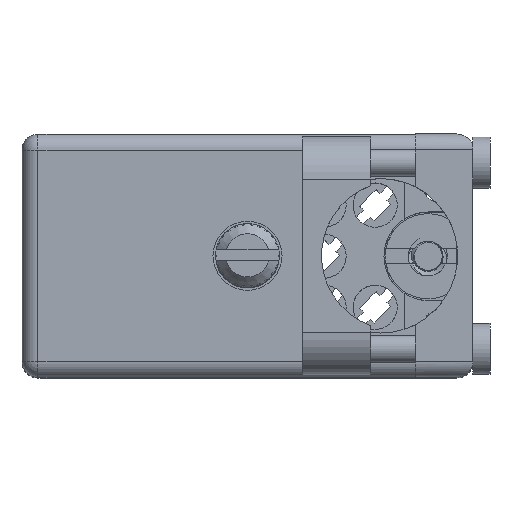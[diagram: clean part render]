
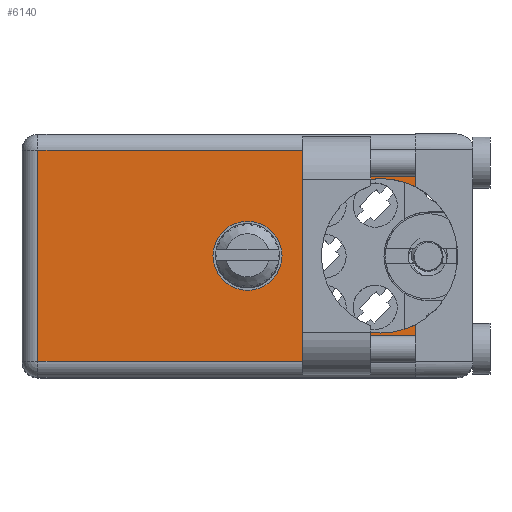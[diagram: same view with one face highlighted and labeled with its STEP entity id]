
A CAD part, top view. The second image highlights one B-rep face of the part: STEP entity #6140.
In plain terms, the highlighted face is planar.
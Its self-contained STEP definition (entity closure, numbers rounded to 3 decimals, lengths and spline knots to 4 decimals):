
#1136 = CARTESIAN_POINT ( 'NONE',  ( 1.053, 0.906, -0.3575 ) ) ;
#6140 = ADVANCED_FACE ( 'NONE', ( #109028, #7195 ), #143802, .T. ) ;
#7195 = FACE_BOUND ( 'NONE', #37577, .T. ) ;
#7939 = EDGE_CURVE ( 'NONE', #183258, #33568, #13675, .T. ) ;
#9528 = VERTEX_POINT ( 'NONE', #151142 ) ;
#9770 = DIRECTION ( 'NONE',  ( 0., 0., 1. ) ) ;
#9917 = DIRECTION ( 'NONE',  ( 0., 0., 1. ) ) ;
#13675 = CIRCLE ( 'NONE', #28924, 0.227 ) ;
#15216 = LINE ( 'NONE', #37053, #128751 ) ;
#16511 = CARTESIAN_POINT ( 'NONE',  ( 1.155, 0.906, -0.047 ) ) ;
#20116 = CIRCLE ( 'NONE', #103181, 0.1015 ) ;
#27319 = CARTESIAN_POINT ( 'NONE',  ( 1.053, 0.906, -0.3575 ) ) ;
#27502 = VERTEX_POINT ( 'NONE', #127699 ) ;
#28924 = AXIS2_PLACEMENT_3D ( 'NONE', #80984, #184537, #99670 ) ;
#32503 = VECTOR ( 'NONE', #9917, 39.3701 ) ;
#33568 = VERTEX_POINT ( 'NONE', #42407 ) ;
#33758 = VERTEX_POINT ( 'NONE', #16511 ) ;
#36084 = CARTESIAN_POINT ( 'NONE',  ( 1.155, 0.906, 0. ) ) ;
#37053 = CARTESIAN_POINT ( 'NONE',  ( 1.155, 0.906, -0.047 ) ) ;
#37577 = EDGE_LOOP ( 'NONE', ( #189435, #42426 ) ) ;
#41265 = VERTEX_POINT ( 'NONE', #84874 ) ;
#41663 = CIRCLE ( 'NONE', #69312, 0.1015 ) ;
#42241 = DIRECTION ( 'NONE',  ( 0., 0., 1. ) ) ;
#42407 = CARTESIAN_POINT ( 'NONE',  ( 1.053, 0.906, -0.1305 ) ) ;
#42426 = ORIENTED_EDGE ( 'NONE', *, *, #114683, .F. ) ;
#43009 = ORIENTED_EDGE ( 'NONE', *, *, #78092, .F. ) ;
#52280 = CARTESIAN_POINT ( 'NONE',  ( 0.6625, 0.906, -0.3575 ) ) ;
#53597 = AXIS2_PLACEMENT_3D ( 'NONE', #1136, #150107, #147504 ) ;
#53755 = VECTOR ( 'NONE', #184150, 39.3701 ) ;
#53814 = ORIENTED_EDGE ( 'NONE', *, *, #183265, .F. ) ;
#54839 = DIRECTION ( 'NONE',  ( 0., 1., 0. ) ) ;
#57196 = DIRECTION ( 'NONE',  ( 0., 1., 0. ) ) ;
#58716 = ORIENTED_EDGE ( 'NONE', *, *, #7939, .F. ) ;
#62073 = CARTESIAN_POINT ( 'NONE',  ( 1.053, 0.906, -0.5845 ) ) ;
#63415 = VERTEX_POINT ( 'NONE', #100840 ) ;
#65922 = AXIS2_PLACEMENT_3D ( 'NONE', #158731, #141915, #9770 ) ;
#69312 = AXIS2_PLACEMENT_3D ( 'NONE', #100606, #57196, #98710 ) ;
#78092 = EDGE_CURVE ( 'NONE', #116391, #183258, #175600, .T. ) ;
#80984 = CARTESIAN_POINT ( 'NONE',  ( 1.053, 0.906, -0.3575 ) ) ;
#81599 = EDGE_CURVE ( 'NONE', #63415, #41265, #140386, .T. ) ;
#84874 = CARTESIAN_POINT ( 'NONE',  ( 0.047, 0.906, -0.047 ) ) ;
#90795 = ORIENTED_EDGE ( 'NONE', *, *, #81599, .T. ) ;
#94209 = CARTESIAN_POINT ( 'NONE',  ( 0., 0.906, -0.668 ) ) ;
#98710 = DIRECTION ( 'NONE',  ( 0., 0., 1. ) ) ;
#99670 = DIRECTION ( 'NONE',  ( 0., 0., 1. ) ) ;
#100606 = CARTESIAN_POINT ( 'NONE',  ( 0.6625, 0.906, -0.3575 ) ) ;
#100840 = CARTESIAN_POINT ( 'NONE',  ( 0.047, 0.906, -0.668 ) ) ;
#103181 = AXIS2_PLACEMENT_3D ( 'NONE', #52280, #54839, #158448 ) ;
#107796 = EDGE_CURVE ( 'NONE', #9528, #63415, #183462, .T. ) ;
#109028 = FACE_OUTER_BOUND ( 'NONE', #133324, .T. ) ;
#112223 = VERTEX_POINT ( 'NONE', #140063 ) ;
#114683 = EDGE_CURVE ( 'NONE', #27502, #186043, #20116, .T. ) ;
#116391 = VERTEX_POINT ( 'NONE', #187003 ) ;
#119215 = EDGE_CURVE ( 'NONE', #186043, #27502, #41663, .T. ) ;
#120023 = VECTOR ( 'NONE', #153345, 39.3701 ) ;
#125091 = EDGE_CURVE ( 'NONE', #41265, #33758, #15216, .T. ) ;
#126519 = AXIS2_PLACEMENT_3D ( 'NONE', #27319, #130902, #42241 ) ;
#127699 = CARTESIAN_POINT ( 'NONE',  ( 0.6625, 0.906, -0.459 ) ) ;
#128741 = CARTESIAN_POINT ( 'NONE',  ( 0.047, 0.906, -0.715 ) ) ;
#128751 = VECTOR ( 'NONE', #140657, 39.3701 ) ;
#130902 = DIRECTION ( 'NONE',  ( 0., 1., 0. ) ) ;
#133324 = EDGE_LOOP ( 'NONE', ( #53814, #171525, #90795, #149166, #173152, #147024, #58716, #43009 ) ) ;
#133467 = VECTOR ( 'NONE', #146830, 39.3701 ) ;
#140063 = CARTESIAN_POINT ( 'NONE',  ( 1.155, 0.906, -0.1547 ) ) ;
#140153 = CARTESIAN_POINT ( 'NONE',  ( 1.155, 0.906, 0. ) ) ;
#140386 = LINE ( 'NONE', #128741, #133467 ) ;
#140657 = DIRECTION ( 'NONE',  ( 1., 0., 0. ) ) ;
#141915 = DIRECTION ( 'NONE',  ( 0., 1., 0. ) ) ;
#143600 = EDGE_CURVE ( 'NONE', #112223, #33758, #166810, .T. ) ;
#143802 = PLANE ( 'NONE',  #65922 ) ;
#146830 = DIRECTION ( 'NONE',  ( 0., 0., 1. ) ) ;
#147024 = ORIENTED_EDGE ( 'NONE', *, *, #173119, .F. ) ;
#147504 = DIRECTION ( 'NONE',  ( 0., 0., 1. ) ) ;
#149166 = ORIENTED_EDGE ( 'NONE', *, *, #125091, .T. ) ;
#150107 = DIRECTION ( 'NONE',  ( 0., 1., 0. ) ) ;
#151142 = CARTESIAN_POINT ( 'NONE',  ( 1.155, 0.906, -0.668 ) ) ;
#153345 = DIRECTION ( 'NONE',  ( 0., 0., 1. ) ) ;
#158448 = DIRECTION ( 'NONE',  ( 0., 0., 1. ) ) ;
#158731 = CARTESIAN_POINT ( 'NONE',  ( 0., 0.906, -0.715 ) ) ;
#159467 = LINE ( 'NONE', #36084, #120023 ) ;
#166810 = LINE ( 'NONE', #140153, #32503 ) ;
#171525 = ORIENTED_EDGE ( 'NONE', *, *, #107796, .T. ) ;
#173119 = EDGE_CURVE ( 'NONE', #33568, #112223, #184312, .T. ) ;
#173152 = ORIENTED_EDGE ( 'NONE', *, *, #143600, .F. ) ;
#175600 = CIRCLE ( 'NONE', #53597, 0.227 ) ;
#183258 = VERTEX_POINT ( 'NONE', #62073 ) ;
#183265 = EDGE_CURVE ( 'NONE', #9528, #116391, #159467, .T. ) ;
#183462 = LINE ( 'NONE', #94209, #53755 ) ;
#184150 = DIRECTION ( 'NONE',  ( -1., 0., 0. ) ) ;
#184312 = CIRCLE ( 'NONE', #126519, 0.227 ) ;
#184537 = DIRECTION ( 'NONE',  ( 0., 1., 0. ) ) ;
#186043 = VERTEX_POINT ( 'NONE', #187924 ) ;
#187003 = CARTESIAN_POINT ( 'NONE',  ( 1.155, 0.906, -0.5603 ) ) ;
#187924 = CARTESIAN_POINT ( 'NONE',  ( 0.6625, 0.906, -0.256 ) ) ;
#189435 = ORIENTED_EDGE ( 'NONE', *, *, #119215, .F. ) ;
